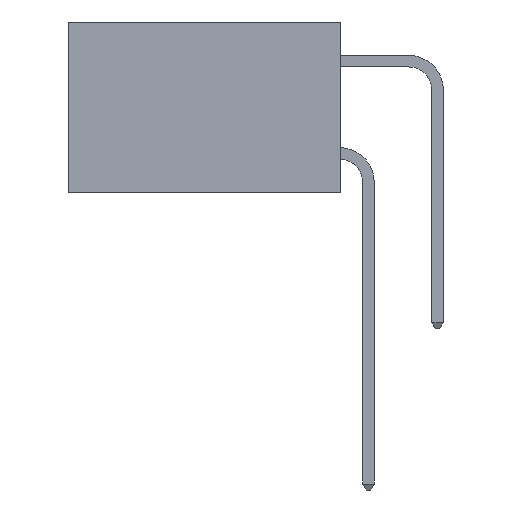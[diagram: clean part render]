
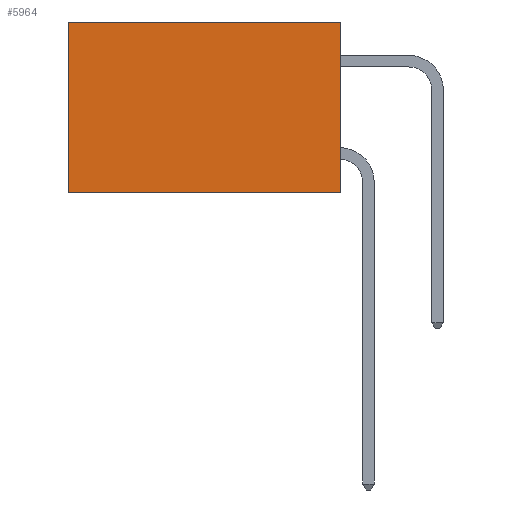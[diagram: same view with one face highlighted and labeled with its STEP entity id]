
A CAD part, left-side view. The second image highlights one B-rep face of the part: STEP entity #5964.
In plain terms, the highlighted planar face has unit normal (-1, 0, 0).
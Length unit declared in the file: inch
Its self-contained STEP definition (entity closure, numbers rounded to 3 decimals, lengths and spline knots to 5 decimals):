
#3 = DIRECTION ( 'NONE',  ( 0., 1., 0. ) ) ;
#76 = CARTESIAN_POINT ( 'NONE',  ( 0.277, 0., -0.37 ) ) ;
#323 = EDGE_CURVE ( 'NONE', #10861, #3225, #429, .T. ) ;
#429 = LINE ( 'NONE', #5321, #4815 ) ;
#449 = ORIENTED_EDGE ( 'NONE', *, *, #323, .T. ) ;
#479 = FACE_OUTER_BOUND ( 'NONE', #2058, .T. ) ;
#604 = CARTESIAN_POINT ( 'NONE',  ( 0.277, 0., -0.37 ) ) ;
#900 = EDGE_CURVE ( 'NONE', #9467, #6351, #1929, .T. ) ;
#961 = ORIENTED_EDGE ( 'NONE', *, *, #7742, .F. ) ;
#1181 = DIRECTION ( 'NONE',  ( 0., 1., 0. ) ) ;
#1702 = DIRECTION ( 'NONE',  ( 0., 0., -1. ) ) ;
#1929 = LINE ( 'NONE', #604, #8895 ) ;
#2058 = EDGE_LOOP ( 'NONE', ( #449, #961, #2592, #2604 ) ) ;
#2059 = CARTESIAN_POINT ( 'NONE',  ( 0.277, 0.59, 0. ) ) ;
#2080 = CARTESIAN_POINT ( 'NONE',  ( 0.277, 0., -0.37 ) ) ;
#2403 = VECTOR ( 'NONE', #3, 39.37008 ) ;
#2592 = ORIENTED_EDGE ( 'NONE', *, *, #900, .F. ) ;
#2604 = ORIENTED_EDGE ( 'NONE', *, *, #10855, .T. ) ;
#3019 = CARTESIAN_POINT ( 'NONE',  ( 0.277, 0., 0. ) ) ;
#3225 = VERTEX_POINT ( 'NONE', #5044 ) ;
#4561 = AXIS2_PLACEMENT_3D ( 'NONE', #5138, #5083, #5070 ) ;
#4815 = VECTOR ( 'NONE', #1702, 39.37008 ) ;
#5044 = CARTESIAN_POINT ( 'NONE',  ( 0.277, 0.59, -0.37 ) ) ;
#5070 = DIRECTION ( 'NONE',  ( 0., 0., -1. ) ) ;
#5083 = DIRECTION ( 'NONE',  ( 1., 0., 0. ) ) ;
#5106 = PLANE ( 'NONE',  #4561 ) ;
#5138 = CARTESIAN_POINT ( 'NONE',  ( 0.277, 0., -0.37 ) ) ;
#5321 = CARTESIAN_POINT ( 'NONE',  ( 0.277, 0.59, -0.37 ) ) ;
#5964 = ADVANCED_FACE ( 'NONE', ( #479 ), #5106, .F. ) ;
#6031 = VECTOR ( 'NONE', #1181, 39.37008 ) ;
#6351 = VERTEX_POINT ( 'NONE', #2080 ) ;
#7742 = EDGE_CURVE ( 'NONE', #6351, #3225, #9048, .T. ) ;
#8071 = DIRECTION ( 'NONE',  ( 0., 0., -1. ) ) ;
#8895 = VECTOR ( 'NONE', #8071, 39.37008 ) ;
#9048 = LINE ( 'NONE', #76, #2403 ) ;
#9467 = VERTEX_POINT ( 'NONE', #3019 ) ;
#10386 = CARTESIAN_POINT ( 'NONE',  ( 0.277, 0., 0. ) ) ;
#10633 = LINE ( 'NONE', #10386, #6031 ) ;
#10855 = EDGE_CURVE ( 'NONE', #9467, #10861, #10633, .T. ) ;
#10861 = VERTEX_POINT ( 'NONE', #2059 ) ;
